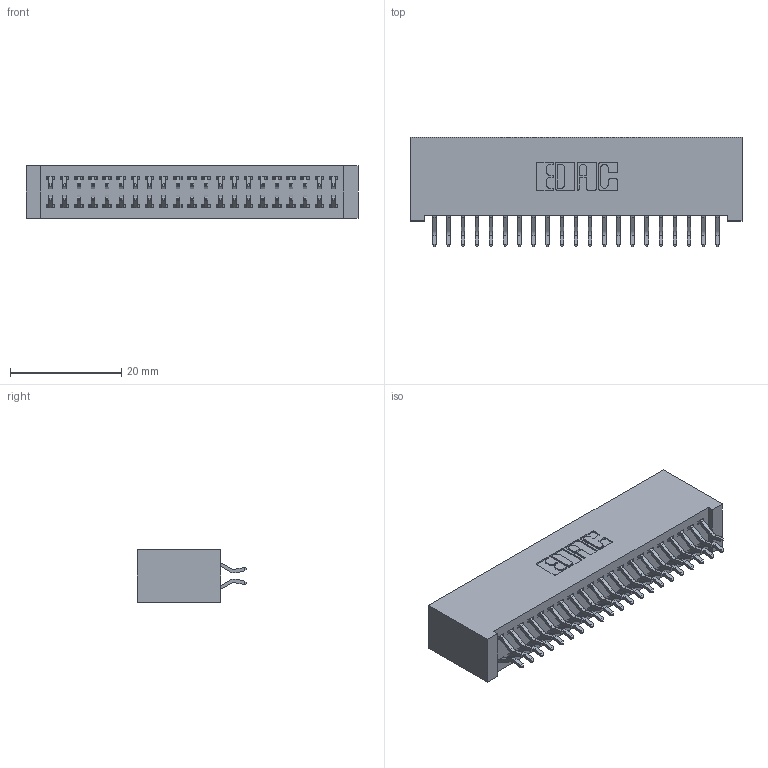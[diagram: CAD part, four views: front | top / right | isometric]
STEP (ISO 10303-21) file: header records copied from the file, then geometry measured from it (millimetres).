
FILE_DESCRIPTION (( 'STEP AP203' ), '1' );
FILE_NAME ('342-042-556-201.STEP', '2018-08-12T13:20:31', ( '' ), ( '' ), 'SwSTEP 2.0', 'SolidWorks 2016', '' );
FILE_SCHEMA (( 'CONFIG_CONTROL_DESIGN' ));
Length unit declared in the file: inch
Products named in the file (3): 342 Part_Lugless; 345-292-001_556 Tail; 342-042-556-201
Assembly tree (43 placements, depth 2):
  342-042-556-201
    342 Part_Lugless
    345-292-001_556 Tail  x42
Bounding box: 59.59 x 19.58 x 9.4 mm (x, y, z)
Volume: 5693.1 mm3; surface area: 9154.9 mm2
Topology: 43 solids, 43 shells, 2538 faces, 7541 edges, 4970 vertices
Faces by surface type: plane 1742, cylinder 796
Entity records: 16037 total; most frequent: CARTESIAN_POINT 2694, ORIENTED_EDGE 2618, DIRECTION 2321, EDGE_CURVE 1309, LINE 1181, VECTOR 1181, VERTEX_POINT 870, AXIS2_PLACEMENT_3D 570
